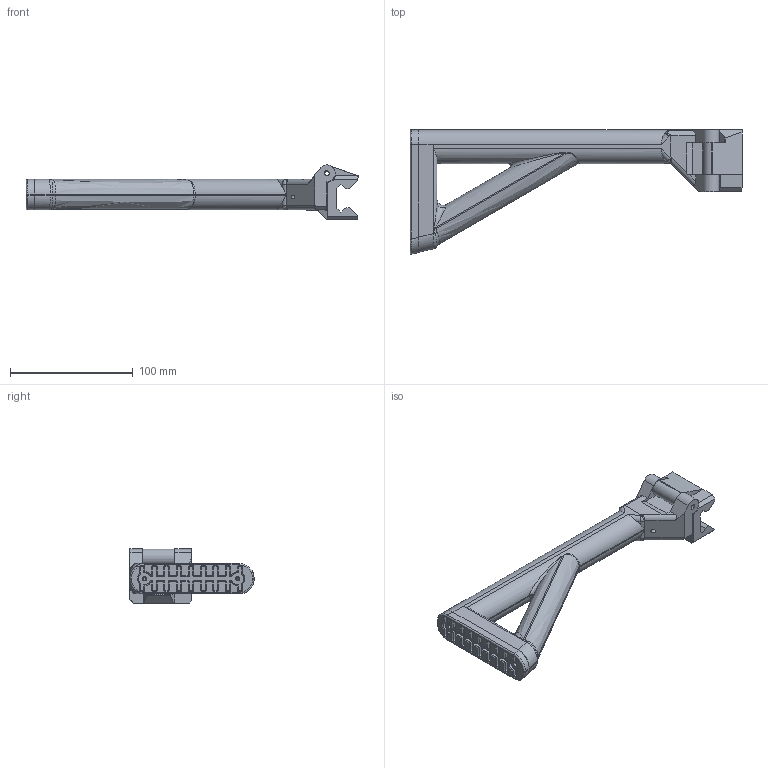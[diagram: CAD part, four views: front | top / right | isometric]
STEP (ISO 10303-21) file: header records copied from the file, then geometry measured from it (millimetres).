
FILE_DESCRIPTION(/* description */ (''),/* implementation_level */ '2;1');
FILE_NAME(/* name */ 'PDW Stock x.stp',/* time_stamp */ '2021-01-17T16:38:21+02:00',/* author */ (''),/* organization */ (''),/* preprocessor_version */ 'ST-DEVELOPER v15.2',/* originating_system */ 'Autodesk Translator Framework v2.0.0.5431',/* authorisation */ '');
FILE_SCHEMA (('AUTOMOTIVE_DESIGN { 1 0 10303 214 3 1 1 }'));
Length unit declared in the file: centimetre
Products named in the file (1): (Unsaved)
Bounding box: 270.92 x 101.42 x 44.3 mm (x, y, z)
Volume: 216972.5 mm3; surface area: 75882.5 mm2
Topology: 4 solids, 4 shells, 521 faces, 1329 edges, 818 vertices
Faces by surface type: plane 268, cylinder 140, cone 71, bspline 38, torus 4
Full cylindrical faces by diameter (mm): 2.5 x2, 3 x1, 3.5 x2, 4 x3, 12.1 x1, 20.5 x1
Entity records: 18525 total; most frequent: CARTESIAN_POINT 5943, ORIENTED_EDGE 2630, DIRECTION 2606, EDGE_CURVE 1314, AXIS2_PLACEMENT_3D 875, LINE 856, VECTOR 856, VERTEX_POINT 814
